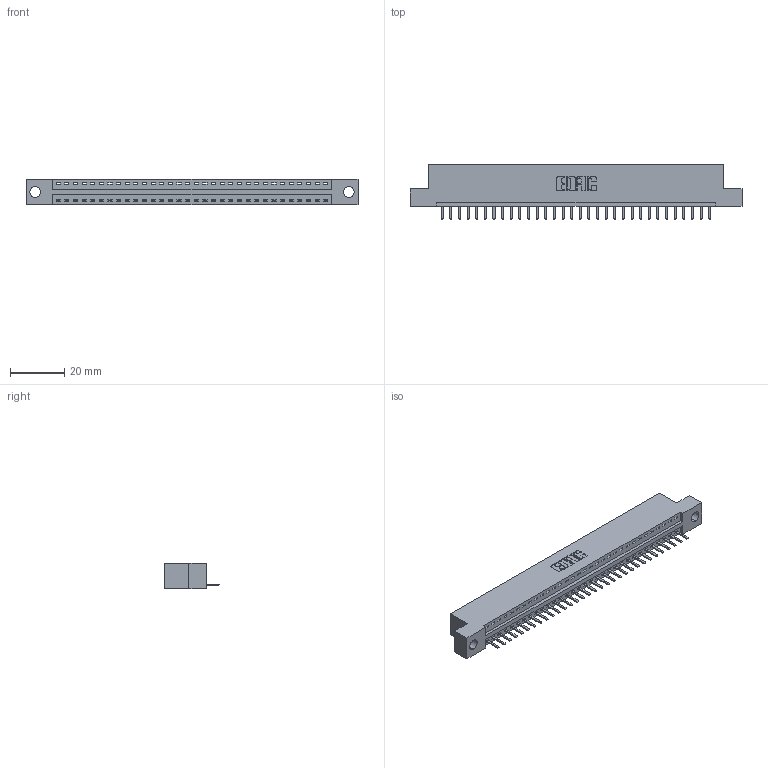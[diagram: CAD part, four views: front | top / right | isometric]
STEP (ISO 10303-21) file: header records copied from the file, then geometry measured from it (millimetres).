
FILE_DESCRIPTION (( 'STEP AP203' ), '1' );
FILE_NAME ('346-032-520-104.STEP', '2022-05-06T17:50:05', ( '' ), ( '' ), 'SwSTEP 2.0', 'SolidWorks 2020', '' );
FILE_SCHEMA (( 'CONFIG_CONTROL_DESIGN' ));
Length unit declared in the file: inch
Products named in the file (3): 346 Part_Flush Mounting Lugs - 0.156 Dia-TH; 346-032-520-104; 345-292-001_345-293-120
Assembly tree (33 placements, depth 2):
  346-032-520-104
    346 Part_Flush Mounting Lugs - 0.156 Dia-TH
    345-292-001_345-293-120  x32
Bounding box: 122.17 x 20.02 x 9.4 mm (x, y, z)
Volume: 11427.9 mm3; surface area: 13705.4 mm2
Topology: 33 solids, 33 shells, 2120 faces, 6253 edges, 4082 vertices
Faces by surface type: plane 1434, cylinder 686
Entity records: 21739 total; most frequent: CARTESIAN_POINT 3750, ORIENTED_EDGE 3702, DIRECTION 3307, EDGE_CURVE 1851, VECTOR 1587, LINE 1587, VERTEX_POINT 1230, AXIS2_PLACEMENT_3D 860
